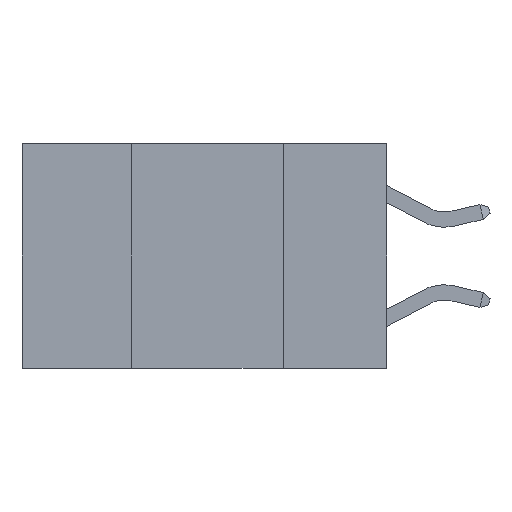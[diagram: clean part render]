
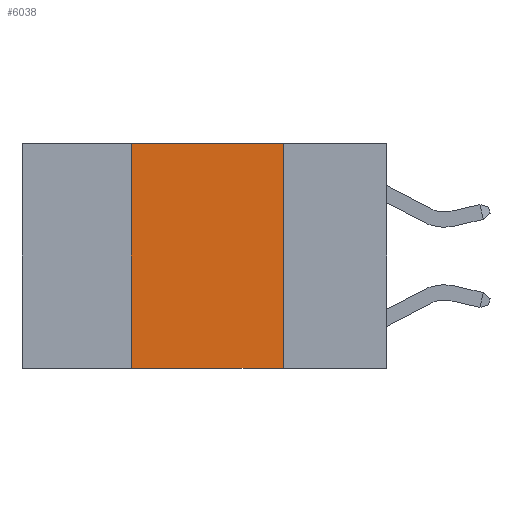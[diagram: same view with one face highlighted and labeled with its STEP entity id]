
A CAD part, left-side view. The second image highlights one B-rep face of the part: STEP entity #6038.
In plain terms, the highlighted planar face has unit normal (-1, 0, 0).
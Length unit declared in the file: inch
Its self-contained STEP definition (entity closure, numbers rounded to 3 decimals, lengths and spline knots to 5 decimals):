
#355 = DIRECTION ( 'NONE',  ( 1., 0., 0. ) ) ;
#565 = PLANE ( 'NONE',  #6478 ) ;
#666 = ORIENTED_EDGE ( 'NONE', *, *, #18412, .F. ) ;
#1591 = VECTOR ( 'NONE', #10445, 39.37008 ) ;
#4067 = EDGE_CURVE ( 'NONE', #10427, #9553, #17716, .T. ) ;
#4318 = LINE ( 'NONE', #15074, #10380 ) ;
#4616 = EDGE_CURVE ( 'NONE', #7427, #9841, #7013, .T. ) ;
#5255 = FACE_OUTER_BOUND ( 'NONE', #15345, .T. ) ;
#5777 = CARTESIAN_POINT ( 'NONE',  ( 0., 0.6, -0.37 ) ) ;
#5861 = ORIENTED_EDGE ( 'NONE', *, *, #18436, .T. ) ;
#6038 = ADVANCED_FACE ( 'NONE', ( #5255 ), #565, .F. ) ;
#6215 = ORIENTED_EDGE ( 'NONE', *, *, #4067, .F. ) ;
#6478 = AXIS2_PLACEMENT_3D ( 'NONE', #6822, #355, #6614 ) ;
#6614 = DIRECTION ( 'NONE',  ( 0., 0., -1. ) ) ;
#6822 = CARTESIAN_POINT ( 'NONE',  ( 0., 0.6, 0. ) ) ;
#7013 = LINE ( 'NONE', #10044, #7856 ) ;
#7427 = VERTEX_POINT ( 'NONE', #11601 ) ;
#7856 = VECTOR ( 'NONE', #11585, 39.37008 ) ;
#8486 = VECTOR ( 'NONE', #12874, 39.37008 ) ;
#9553 = VERTEX_POINT ( 'NONE', #12832 ) ;
#9841 = VERTEX_POINT ( 'NONE', #14862 ) ;
#10044 = CARTESIAN_POINT ( 'NONE',  ( 0., 0.17, 0. ) ) ;
#10380 = VECTOR ( 'NONE', #13756, 39.37008 ) ;
#10427 = VERTEX_POINT ( 'NONE', #17038 ) ;
#10445 = DIRECTION ( 'NONE',  ( 0., -1., 0. ) ) ;
#11585 = DIRECTION ( 'NONE',  ( 0., 0., -1. ) ) ;
#11601 = CARTESIAN_POINT ( 'NONE',  ( 0., 0.17, 0. ) ) ;
#12832 = CARTESIAN_POINT ( 'NONE',  ( 0., 0.42, 0. ) ) ;
#12874 = DIRECTION ( 'NONE',  ( 0., 0., 1. ) ) ;
#13167 = CARTESIAN_POINT ( 'NONE',  ( 0., 0.42, 0. ) ) ;
#13756 = DIRECTION ( 'NONE',  ( 0., -1., 0. ) ) ;
#14862 = CARTESIAN_POINT ( 'NONE',  ( 0., 0.17, -0.37 ) ) ;
#15074 = CARTESIAN_POINT ( 'NONE',  ( 0., 0.6, 0. ) ) ;
#15345 = EDGE_LOOP ( 'NONE', ( #19161, #666, #6215, #5861 ) ) ;
#17038 = CARTESIAN_POINT ( 'NONE',  ( 0., 0.42, -0.37 ) ) ;
#17716 = LINE ( 'NONE', #13167, #8486 ) ;
#18412 = EDGE_CURVE ( 'NONE', #9553, #7427, #4318, .T. ) ;
#18436 = EDGE_CURVE ( 'NONE', #10427, #9841, #19748, .T. ) ;
#19161 = ORIENTED_EDGE ( 'NONE', *, *, #4616, .F. ) ;
#19748 = LINE ( 'NONE', #5777, #1591 ) ;
